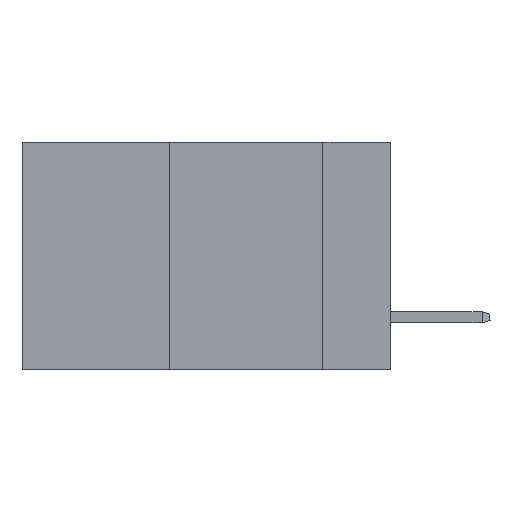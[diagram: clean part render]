
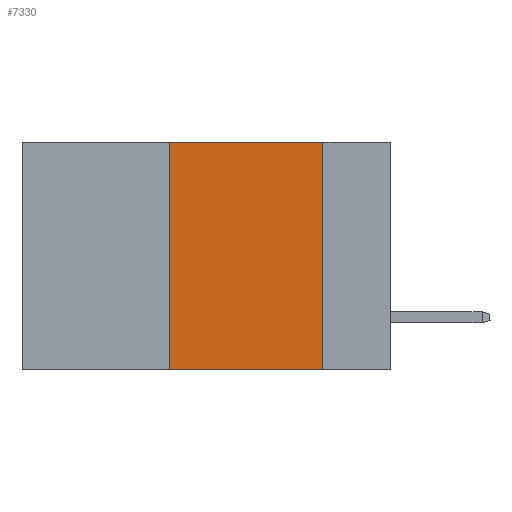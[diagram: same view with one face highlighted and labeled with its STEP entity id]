
A CAD part, left-side view. The second image highlights one B-rep face of the part: STEP entity #7330.
In plain terms, the highlighted planar face has unit normal (-1, 0, 0).
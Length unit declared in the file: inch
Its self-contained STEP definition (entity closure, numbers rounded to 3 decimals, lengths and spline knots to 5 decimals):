
#1174 = CARTESIAN_POINT ( 'NONE',  ( 0., 0.6, 0. ) ) ;
#1345 = EDGE_CURVE ( 'NONE', #11855, #33235, #9012, .T. ) ;
#1419 = ORIENTED_EDGE ( 'NONE', *, *, #9635, .F. ) ;
#1628 = CARTESIAN_POINT ( 'NONE',  ( 0., 0.36, -0.37 ) ) ;
#1684 = LINE ( 'NONE', #10546, #22641 ) ;
#2051 = ORIENTED_EDGE ( 'NONE', *, *, #1345, .F. ) ;
#2973 = EDGE_CURVE ( 'NONE', #33235, #12691, #32053, .T. ) ;
#4229 = VECTOR ( 'NONE', #20053, 39.37008 ) ;
#7010 = VECTOR ( 'NONE', #9516, 39.37008 ) ;
#7138 = CARTESIAN_POINT ( 'NONE',  ( 0., 0.36, 0. ) ) ;
#7330 = ADVANCED_FACE ( 'NONE', ( #35383 ), #21574, .F. ) ;
#9012 = LINE ( 'NONE', #1174, #22695 ) ;
#9516 = DIRECTION ( 'NONE',  ( 0., 0., 1. ) ) ;
#9635 = EDGE_CURVE ( 'NONE', #18224, #11855, #26722, .T. ) ;
#10163 = AXIS2_PLACEMENT_3D ( 'NONE', #32580, #18363, #16198 ) ;
#10546 = CARTESIAN_POINT ( 'NONE',  ( 0., 0.6, -0.37 ) ) ;
#11855 = VERTEX_POINT ( 'NONE', #16896 ) ;
#12105 = EDGE_CURVE ( 'NONE', #18224, #12691, #1684, .T. ) ;
#12574 = ORIENTED_EDGE ( 'NONE', *, *, #2973, .F. ) ;
#12691 = VERTEX_POINT ( 'NONE', #18541 ) ;
#16037 = EDGE_LOOP ( 'NONE', ( #12574, #2051, #1419, #33198 ) ) ;
#16198 = DIRECTION ( 'NONE',  ( 0., 0., -1. ) ) ;
#16896 = CARTESIAN_POINT ( 'NONE',  ( 0., 0.36, 0. ) ) ;
#17833 = DIRECTION ( 'NONE',  ( 0., -1., 0. ) ) ;
#18224 = VERTEX_POINT ( 'NONE', #1628 ) ;
#18363 = DIRECTION ( 'NONE',  ( 1., 0., 0. ) ) ;
#18541 = CARTESIAN_POINT ( 'NONE',  ( 0., 0.11, -0.37 ) ) ;
#20053 = DIRECTION ( 'NONE',  ( 0., 0., -1. ) ) ;
#21574 = PLANE ( 'NONE',  #10163 ) ;
#22641 = VECTOR ( 'NONE', #32315, 39.37008 ) ;
#22695 = VECTOR ( 'NONE', #17833, 39.37008 ) ;
#25896 = CARTESIAN_POINT ( 'NONE',  ( 0., 0.11, 0. ) ) ;
#26722 = LINE ( 'NONE', #7138, #7010 ) ;
#27594 = CARTESIAN_POINT ( 'NONE',  ( 0., 0.11, 0. ) ) ;
#32053 = LINE ( 'NONE', #27594, #4229 ) ;
#32315 = DIRECTION ( 'NONE',  ( 0., -1., 0. ) ) ;
#32580 = CARTESIAN_POINT ( 'NONE',  ( 0., 0.6, 0. ) ) ;
#33198 = ORIENTED_EDGE ( 'NONE', *, *, #12105, .T. ) ;
#33235 = VERTEX_POINT ( 'NONE', #25896 ) ;
#35383 = FACE_OUTER_BOUND ( 'NONE', #16037, .T. ) ;
